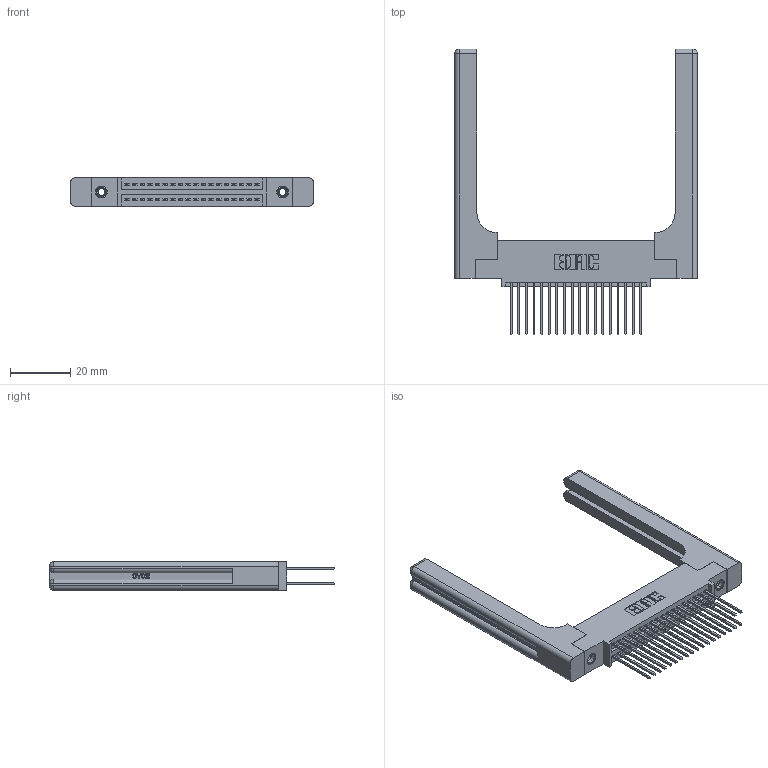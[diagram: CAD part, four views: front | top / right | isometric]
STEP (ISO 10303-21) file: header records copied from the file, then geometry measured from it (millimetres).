
FILE_DESCRIPTION (( 'STEP AP203' ), '1' );
FILE_NAME ('345-036-542-558.STEP', '2019-10-28T12:17:34', ( '' ), ( '' ), 'SwSTEP 2.0', 'SolidWorks 2016', '' );
FILE_SCHEMA (( 'CONFIG_CONTROL_DESIGN' ));
Length unit declared in the file: inch
Products named in the file (5): 345-220-058_345-220-058; 345-292-001_345-293-142; 345-250-001_345-250-001-102; 345 Part_0.110 Offset - 0.156 Dia-TH; 345-036-542-558
Assembly tree (41 placements, depth 2):
  345-036-542-558
    345 Part_0.110 Offset - 0.156 Dia-TH
    345-292-001_345-293-142  x36
    345-250-001_345-250-001-102  x2
    345-220-058_345-220-058  x2
Bounding box: 80.75 x 95.05 x 9.4 mm (x, y, z)
Volume: 16190.6 mm3; surface area: 16875.9 mm2
Topology: 41 solids, 41 shells, 2186 faces, 6383 edges, 4186 vertices
Faces by surface type: plane 1420, cylinder 706, bspline 36, cone 12, sphere 8, torus 4
Entity records: 22686 total; most frequent: CARTESIAN_POINT 4821, ORIENTED_EDGE 3552, DIRECTION 3212, EDGE_CURVE 1776, VECTOR 1480, LINE 1480, VERTEX_POINT 1174, AXIS2_PLACEMENT_3D 866
